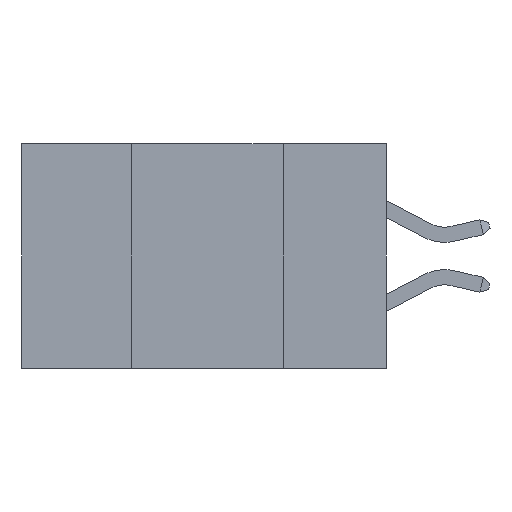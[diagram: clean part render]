
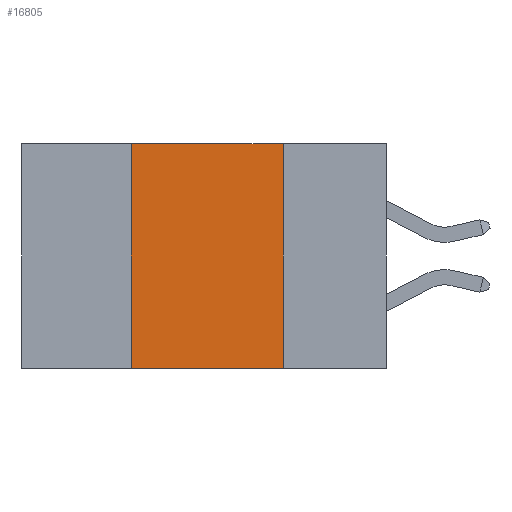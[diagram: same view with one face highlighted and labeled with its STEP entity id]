
A CAD part, left-side view. The second image highlights one B-rep face of the part: STEP entity #16805.
In plain terms, the highlighted planar face has unit normal (-1, 0, 0).
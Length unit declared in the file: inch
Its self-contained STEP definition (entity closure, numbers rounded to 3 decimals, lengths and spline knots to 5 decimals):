
#84 = DIRECTION ( 'NONE',  ( 1., 0., 0. ) ) ;
#621 = EDGE_CURVE ( 'NONE', #13956, #17798, #14911, .T. ) ;
#1114 = DIRECTION ( 'NONE',  ( 0., -1., 0. ) ) ;
#1250 = LINE ( 'NONE', #4074, #1701 ) ;
#1701 = VECTOR ( 'NONE', #14116, 39.37008 ) ;
#3045 = DIRECTION ( 'NONE',  ( 0., 0., 1. ) ) ;
#3136 = VERTEX_POINT ( 'NONE', #9729 ) ;
#3198 = ORIENTED_EDGE ( 'NONE', *, *, #12750, .T. ) ;
#3861 = VECTOR ( 'NONE', #12907, 39.37008 ) ;
#3905 = EDGE_CURVE ( 'NONE', #17798, #10239, #1250, .T. ) ;
#4074 = CARTESIAN_POINT ( 'NONE',  ( 0., 0.17, 0. ) ) ;
#4293 = ORIENTED_EDGE ( 'NONE', *, *, #13936, .F. ) ;
#5830 = CARTESIAN_POINT ( 'NONE',  ( 0., 0.6, 0. ) ) ;
#6691 = EDGE_LOOP ( 'NONE', ( #10089, #16408, #4293, #3198 ) ) ;
#7352 = PLANE ( 'NONE',  #16793 ) ;
#7998 = CARTESIAN_POINT ( 'NONE',  ( 0., 0.6, 0. ) ) ;
#8753 = CARTESIAN_POINT ( 'NONE',  ( 0., 0.42, 0. ) ) ;
#9729 = CARTESIAN_POINT ( 'NONE',  ( 0., 0.42, -0.37 ) ) ;
#9851 = VECTOR ( 'NONE', #1114, 39.37008 ) ;
#10089 = ORIENTED_EDGE ( 'NONE', *, *, #3905, .F. ) ;
#10239 = VERTEX_POINT ( 'NONE', #17366 ) ;
#10282 = DIRECTION ( 'NONE',  ( 0., 0., -1. ) ) ;
#12001 = FACE_OUTER_BOUND ( 'NONE', #6691, .T. ) ;
#12531 = VECTOR ( 'NONE', #3045, 39.37008 ) ;
#12750 = EDGE_CURVE ( 'NONE', #3136, #10239, #17441, .T. ) ;
#12907 = DIRECTION ( 'NONE',  ( 0., -1., 0. ) ) ;
#13747 = CARTESIAN_POINT ( 'NONE',  ( 0., 0.17, 0. ) ) ;
#13936 = EDGE_CURVE ( 'NONE', #3136, #13956, #16746, .T. ) ;
#13956 = VERTEX_POINT ( 'NONE', #16001 ) ;
#14116 = DIRECTION ( 'NONE',  ( 0., 0., -1. ) ) ;
#14911 = LINE ( 'NONE', #7998, #3861 ) ;
#16001 = CARTESIAN_POINT ( 'NONE',  ( 0., 0.42, 0. ) ) ;
#16408 = ORIENTED_EDGE ( 'NONE', *, *, #621, .F. ) ;
#16746 = LINE ( 'NONE', #8753, #12531 ) ;
#16793 = AXIS2_PLACEMENT_3D ( 'NONE', #5830, #84, #10282 ) ;
#16805 = ADVANCED_FACE ( 'NONE', ( #12001 ), #7352, .F. ) ;
#16989 = CARTESIAN_POINT ( 'NONE',  ( 0., 0.6, -0.37 ) ) ;
#17366 = CARTESIAN_POINT ( 'NONE',  ( 0., 0.17, -0.37 ) ) ;
#17441 = LINE ( 'NONE', #16989, #9851 ) ;
#17798 = VERTEX_POINT ( 'NONE', #13747 ) ;
